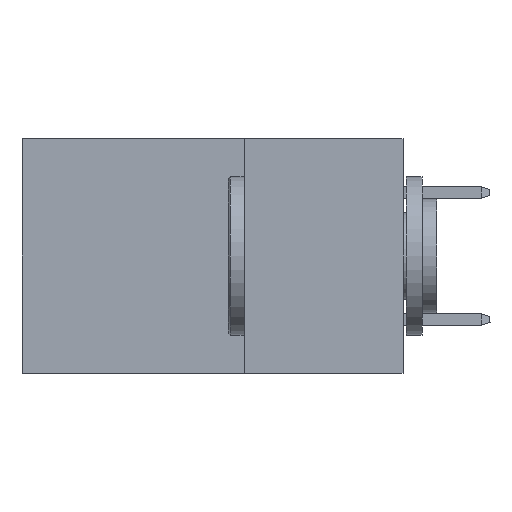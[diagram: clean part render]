
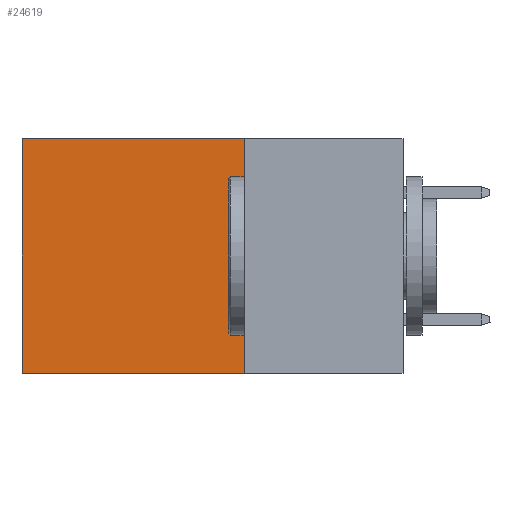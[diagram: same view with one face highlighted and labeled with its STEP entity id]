
A CAD part, left-side view. The second image highlights one B-rep face of the part: STEP entity #24619.
In plain terms, the highlighted planar face has unit normal (-1, 0, 0).
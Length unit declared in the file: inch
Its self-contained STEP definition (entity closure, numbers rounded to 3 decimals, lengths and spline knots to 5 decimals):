
#208 = ORIENTED_EDGE ( 'NONE', *, *, #5822, .T. ) ;
#2848 = LINE ( 'NONE', #5361, #28082 ) ;
#4698 = CARTESIAN_POINT ( 'NONE',  ( 0.2875, 0.25, 0. ) ) ;
#5361 = CARTESIAN_POINT ( 'NONE',  ( 0.2875, 0.25, -0.37 ) ) ;
#5362 = CARTESIAN_POINT ( 'NONE',  ( 0.2875, 0.6, 0. ) ) ;
#5647 = CARTESIAN_POINT ( 'NONE',  ( 0.2875, 0.25, 0. ) ) ;
#5822 = EDGE_CURVE ( 'NONE', #13791, #23561, #25647, .T. ) ;
#5863 = EDGE_CURVE ( 'NONE', #9531, #23112, #2848, .T. ) ;
#6680 = VECTOR ( 'NONE', #20588, 39.37008 ) ;
#7743 = ORIENTED_EDGE ( 'NONE', *, *, #7868, .T. ) ;
#7868 = EDGE_CURVE ( 'NONE', #23561, #23112, #23421, .T. ) ;
#8881 = ORIENTED_EDGE ( 'NONE', *, *, #19544, .F. ) ;
#9531 = VERTEX_POINT ( 'NONE', #9712 ) ;
#9712 = CARTESIAN_POINT ( 'NONE',  ( 0.2875, 0.25, -0.37 ) ) ;
#10056 = LINE ( 'NONE', #4698, #31849 ) ;
#11372 = PLANE ( 'NONE',  #28840 ) ;
#13081 = DIRECTION ( 'NONE',  ( 0., 1., 0. ) ) ;
#13308 = VECTOR ( 'NONE', #23255, 39.37008 ) ;
#13408 = CARTESIAN_POINT ( 'NONE',  ( 0.2875, 0.25, 0. ) ) ;
#13791 = VERTEX_POINT ( 'NONE', #5647 ) ;
#13878 = CARTESIAN_POINT ( 'NONE',  ( 0.2875, 0.25, 0. ) ) ;
#14591 = DIRECTION ( 'NONE',  ( 0., 0., -1. ) ) ;
#18895 = DIRECTION ( 'NONE',  ( 0., 0., -1. ) ) ;
#19544 = EDGE_CURVE ( 'NONE', #13791, #9531, #10056, .T. ) ;
#20588 = DIRECTION ( 'NONE',  ( 0., 1., 0. ) ) ;
#21213 = EDGE_LOOP ( 'NONE', ( #7743, #24365, #8881, #208 ) ) ;
#22445 = CARTESIAN_POINT ( 'NONE',  ( 0.2875, 0.6, -0.37 ) ) ;
#23112 = VERTEX_POINT ( 'NONE', #22445 ) ;
#23255 = DIRECTION ( 'NONE',  ( 0., 0., -1. ) ) ;
#23421 = LINE ( 'NONE', #5362, #13308 ) ;
#23561 = VERTEX_POINT ( 'NONE', #24441 ) ;
#24077 = DIRECTION ( 'NONE',  ( 1., 0., 0. ) ) ;
#24365 = ORIENTED_EDGE ( 'NONE', *, *, #5863, .F. ) ;
#24441 = CARTESIAN_POINT ( 'NONE',  ( 0.2875, 0.6, 0. ) ) ;
#24619 = ADVANCED_FACE ( 'NONE', ( #31639 ), #11372, .F. ) ;
#25647 = LINE ( 'NONE', #13408, #6680 ) ;
#28082 = VECTOR ( 'NONE', #13081, 39.37008 ) ;
#28840 = AXIS2_PLACEMENT_3D ( 'NONE', #13878, #24077, #18895 ) ;
#31639 = FACE_OUTER_BOUND ( 'NONE', #21213, .T. ) ;
#31849 = VECTOR ( 'NONE', #14591, 39.37008 ) ;
